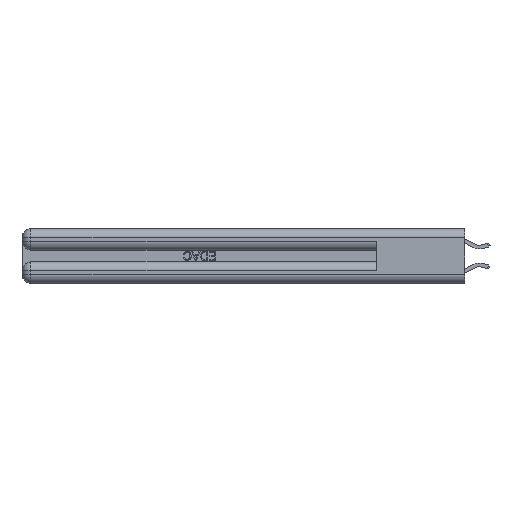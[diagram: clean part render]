
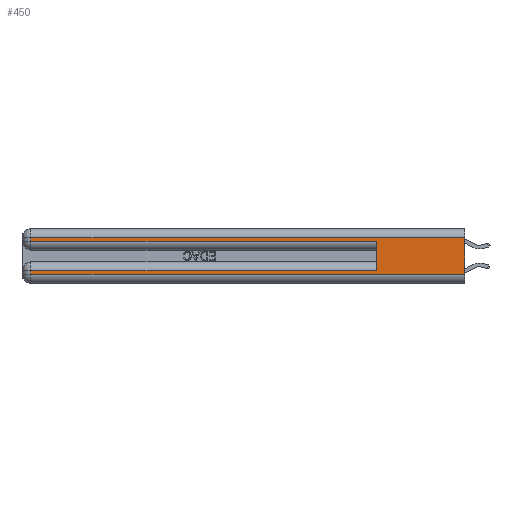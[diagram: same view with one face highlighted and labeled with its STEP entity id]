
A CAD part, left-side view. The second image highlights one B-rep face of the part: STEP entity #450.
In plain terms, the highlighted planar face has unit normal (-1, 0, 0).
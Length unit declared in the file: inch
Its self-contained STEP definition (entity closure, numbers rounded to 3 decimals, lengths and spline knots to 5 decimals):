
#450 = ADVANCED_FACE ( 'NONE', ( #1686 ), #11918, .F. ) ;
#555 = EDGE_CURVE ( 'NONE', #4833, #9798, #14208, .T. ) ;
#980 = DIRECTION ( 'NONE',  ( 0., 0., -1. ) ) ;
#1588 = CARTESIAN_POINT ( 'NONE',  ( 0., 0.6, 0.145 ) ) ;
#1686 = FACE_OUTER_BOUND ( 'NONE', #12283, .T. ) ;
#1751 = DIRECTION ( 'NONE',  ( 0., 0., -1. ) ) ;
#2376 = VERTEX_POINT ( 'NONE', #27247 ) ;
#2952 = CARTESIAN_POINT ( 'NONE',  ( 0., 2.94, 0.37 ) ) ;
#3040 = CARTESIAN_POINT ( 'NONE',  ( 0., 0., 0.085 ) ) ;
#3881 = LINE ( 'NONE', #21340, #10550 ) ;
#4109 = CARTESIAN_POINT ( 'NONE',  ( 0., 0.6, 0.085 ) ) ;
#4343 = ORIENTED_EDGE ( 'NONE', *, *, #31174, .T. ) ;
#4396 = VECTOR ( 'NONE', #19993, 39.37008 ) ;
#4407 = VERTEX_POINT ( 'NONE', #4109 ) ;
#4833 = VERTEX_POINT ( 'NONE', #18354 ) ;
#5681 = CARTESIAN_POINT ( 'NONE',  ( 0., 2.94, 0.085 ) ) ;
#5705 = LINE ( 'NONE', #19160, #31489 ) ;
#6486 = CARTESIAN_POINT ( 'NONE',  ( 0., 0.6, 0.285 ) ) ;
#7493 = VERTEX_POINT ( 'NONE', #20124 ) ;
#9144 = EDGE_CURVE ( 'NONE', #17284, #7493, #10756, .T. ) ;
#9209 = DIRECTION ( 'NONE',  ( 0., 1., 0. ) ) ;
#9627 = CARTESIAN_POINT ( 'NONE',  ( 0., 0., 0.37 ) ) ;
#9798 = VERTEX_POINT ( 'NONE', #6486 ) ;
#10550 = VECTOR ( 'NONE', #1751, 39.37008 ) ;
#10674 = LINE ( 'NONE', #2952, #18099 ) ;
#10724 = LINE ( 'NONE', #16779, #20077 ) ;
#10756 = LINE ( 'NONE', #23830, #29472 ) ;
#11918 = PLANE ( 'NONE',  #22511 ) ;
#11958 = ORIENTED_EDGE ( 'NONE', *, *, #32143, .T. ) ;
#12283 = EDGE_LOOP ( 'NONE', ( #21956, #31880, #28966, #21641, #21408, #4343, #21673, #11958 ) ) ;
#14064 = DIRECTION ( 'NONE',  ( 0., -1., 0. ) ) ;
#14208 = LINE ( 'NONE', #14752, #4396 ) ;
#14611 = CARTESIAN_POINT ( 'NONE',  ( 0., 0., 0.31 ) ) ;
#14752 = CARTESIAN_POINT ( 'NONE',  ( 0., 0., 0.285 ) ) ;
#15471 = LINE ( 'NONE', #3040, #18211 ) ;
#15902 = EDGE_CURVE ( 'NONE', #4407, #9798, #22583, .T. ) ;
#15923 = VECTOR ( 'NONE', #23779, 39.37008 ) ;
#16508 = EDGE_CURVE ( 'NONE', #27530, #2376, #5705, .T. ) ;
#16779 = CARTESIAN_POINT ( 'NONE',  ( 0., 0., 0.06 ) ) ;
#17284 = VERTEX_POINT ( 'NONE', #5681 ) ;
#17402 = CARTESIAN_POINT ( 'NONE',  ( 0., 0., 0.06 ) ) ;
#18099 = VECTOR ( 'NONE', #22971, 39.37008 ) ;
#18211 = VECTOR ( 'NONE', #25343, 39.37008 ) ;
#18354 = CARTESIAN_POINT ( 'NONE',  ( 0., 2.94, 0.285 ) ) ;
#19160 = CARTESIAN_POINT ( 'NONE',  ( 0., 0., 0.31 ) ) ;
#19993 = DIRECTION ( 'NONE',  ( 0., -1., 0. ) ) ;
#20077 = VECTOR ( 'NONE', #14064, 39.37008 ) ;
#20124 = CARTESIAN_POINT ( 'NONE',  ( 0., 2.94, 0.06 ) ) ;
#20248 = EDGE_CURVE ( 'NONE', #27530, #20905, #3881, .T. ) ;
#20905 = VERTEX_POINT ( 'NONE', #17402 ) ;
#21340 = CARTESIAN_POINT ( 'NONE',  ( 0., 0., 0.37 ) ) ;
#21408 = ORIENTED_EDGE ( 'NONE', *, *, #15902, .F. ) ;
#21641 = ORIENTED_EDGE ( 'NONE', *, *, #555, .T. ) ;
#21673 = ORIENTED_EDGE ( 'NONE', *, *, #9144, .T. ) ;
#21956 = ORIENTED_EDGE ( 'NONE', *, *, #20248, .F. ) ;
#22511 = AXIS2_PLACEMENT_3D ( 'NONE', #9627, #27718, #29993 ) ;
#22583 = LINE ( 'NONE', #1588, #15923 ) ;
#22971 = DIRECTION ( 'NONE',  ( 0., 0., -1. ) ) ;
#23779 = DIRECTION ( 'NONE',  ( 0., 0., 1. ) ) ;
#23830 = CARTESIAN_POINT ( 'NONE',  ( 0., 2.94, 0.37 ) ) ;
#25343 = DIRECTION ( 'NONE',  ( 0., 1., 0. ) ) ;
#27247 = CARTESIAN_POINT ( 'NONE',  ( 0., 2.94, 0.31 ) ) ;
#27530 = VERTEX_POINT ( 'NONE', #14611 ) ;
#27633 = EDGE_CURVE ( 'NONE', #2376, #4833, #10674, .T. ) ;
#27718 = DIRECTION ( 'NONE',  ( 1., 0., 0. ) ) ;
#28966 = ORIENTED_EDGE ( 'NONE', *, *, #27633, .T. ) ;
#29472 = VECTOR ( 'NONE', #980, 39.37008 ) ;
#29993 = DIRECTION ( 'NONE',  ( 0., 0., -1. ) ) ;
#31174 = EDGE_CURVE ( 'NONE', #4407, #17284, #15471, .T. ) ;
#31489 = VECTOR ( 'NONE', #9209, 39.37008 ) ;
#31880 = ORIENTED_EDGE ( 'NONE', *, *, #16508, .T. ) ;
#32143 = EDGE_CURVE ( 'NONE', #7493, #20905, #10724, .T. ) ;
